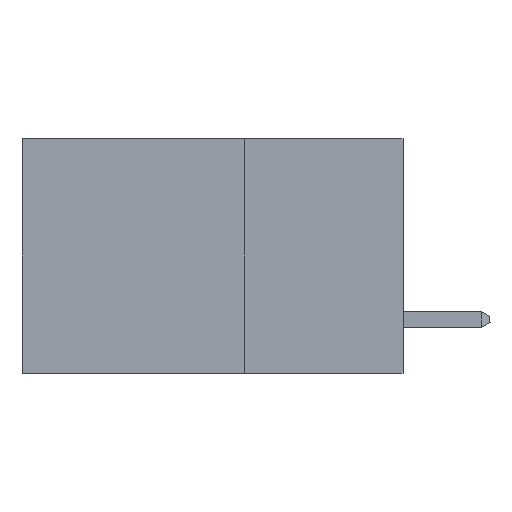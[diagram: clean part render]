
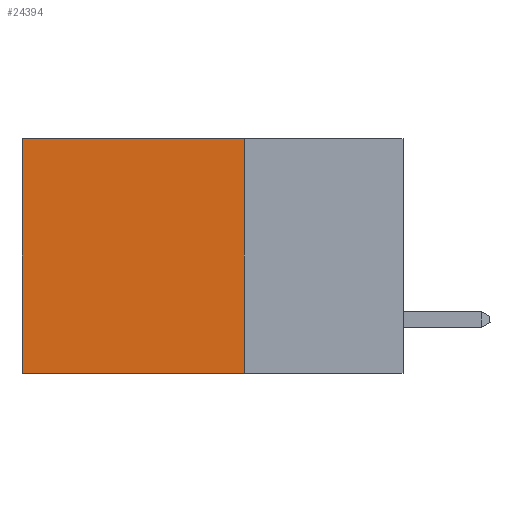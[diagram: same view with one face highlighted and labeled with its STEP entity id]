
A CAD part, left-side view. The second image highlights one B-rep face of the part: STEP entity #24394.
In plain terms, the highlighted planar face has unit normal (-1, 0, 0).
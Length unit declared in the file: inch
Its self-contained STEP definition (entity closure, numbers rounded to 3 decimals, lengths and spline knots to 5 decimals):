
#1234 = PLANE ( 'NONE',  #5174 ) ;
#1300 = CARTESIAN_POINT ( 'NONE',  ( 0.2875, 0.25, 0. ) ) ;
#1467 = VECTOR ( 'NONE', #22121, 39.37008 ) ;
#2103 = VERTEX_POINT ( 'NONE', #15049 ) ;
#2977 = VERTEX_POINT ( 'NONE', #14285 ) ;
#5174 = AXIS2_PLACEMENT_3D ( 'NONE', #19676, #22149, #24423 ) ;
#5290 = VERTEX_POINT ( 'NONE', #10267 ) ;
#5513 = ORIENTED_EDGE ( 'NONE', *, *, #11025, .F. ) ;
#7594 = LINE ( 'NONE', #1300, #1467 ) ;
#9245 = CARTESIAN_POINT ( 'NONE',  ( 0.2875, 0.25, 0. ) ) ;
#10267 = CARTESIAN_POINT ( 'NONE',  ( 0.2875, 0.25, -0.37 ) ) ;
#11025 = EDGE_CURVE ( 'NONE', #5290, #19430, #25419, .T. ) ;
#11194 = VECTOR ( 'NONE', #23091, 39.37008 ) ;
#11612 = DIRECTION ( 'NONE',  ( 0., 0., -1. ) ) ;
#11730 = EDGE_CURVE ( 'NONE', #2103, #19430, #25352, .T. ) ;
#12475 = VECTOR ( 'NONE', #11612, 39.37008 ) ;
#13709 = ORIENTED_EDGE ( 'NONE', *, *, #11730, .T. ) ;
#14073 = EDGE_CURVE ( 'NONE', #2977, #2103, #23432, .T. ) ;
#14285 = CARTESIAN_POINT ( 'NONE',  ( 0.2875, 0.25, 0. ) ) ;
#14960 = ORIENTED_EDGE ( 'NONE', *, *, #22147, .F. ) ;
#15049 = CARTESIAN_POINT ( 'NONE',  ( 0.2875, 0.6, 0. ) ) ;
#17218 = CARTESIAN_POINT ( 'NONE',  ( 0.2875, 0.25, -0.37 ) ) ;
#17969 = VECTOR ( 'NONE', #26272, 39.37008 ) ;
#19018 = CARTESIAN_POINT ( 'NONE',  ( 0.2875, 0.6, -0.37 ) ) ;
#19326 = EDGE_LOOP ( 'NONE', ( #13709, #5513, #14960, #26879 ) ) ;
#19430 = VERTEX_POINT ( 'NONE', #19018 ) ;
#19676 = CARTESIAN_POINT ( 'NONE',  ( 0.2875, 0.25, 0. ) ) ;
#22121 = DIRECTION ( 'NONE',  ( 0., 0., -1. ) ) ;
#22147 = EDGE_CURVE ( 'NONE', #2977, #5290, #7594, .T. ) ;
#22149 = DIRECTION ( 'NONE',  ( 1., 0., 0. ) ) ;
#23091 = DIRECTION ( 'NONE',  ( 0., 1., 0. ) ) ;
#23432 = LINE ( 'NONE', #9245, #11194 ) ;
#24394 = ADVANCED_FACE ( 'NONE', ( #25718 ), #1234, .F. ) ;
#24423 = DIRECTION ( 'NONE',  ( 0., 0., -1. ) ) ;
#24928 = CARTESIAN_POINT ( 'NONE',  ( 0.2875, 0.6, 0. ) ) ;
#25352 = LINE ( 'NONE', #24928, #12475 ) ;
#25419 = LINE ( 'NONE', #17218, #17969 ) ;
#25718 = FACE_OUTER_BOUND ( 'NONE', #19326, .T. ) ;
#26272 = DIRECTION ( 'NONE',  ( 0., 1., 0. ) ) ;
#26879 = ORIENTED_EDGE ( 'NONE', *, *, #14073, .T. ) ;
